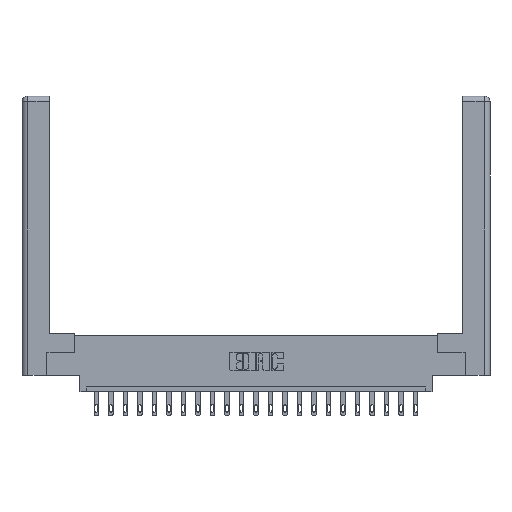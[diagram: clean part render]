
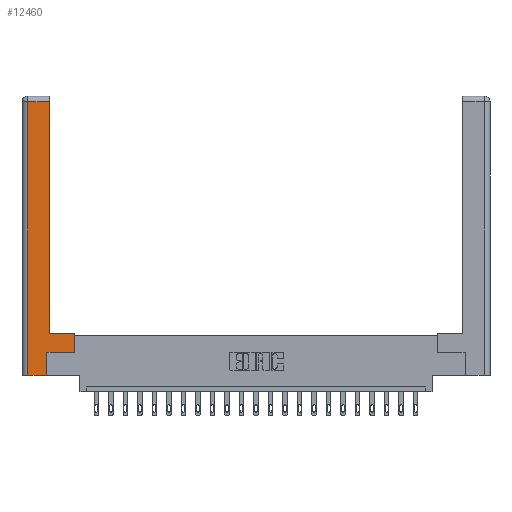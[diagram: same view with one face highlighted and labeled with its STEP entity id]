
A CAD part, top view. The second image highlights one B-rep face of the part: STEP entity #12460.
In plain terms, the highlighted planar face has unit normal (0, 0, 1).
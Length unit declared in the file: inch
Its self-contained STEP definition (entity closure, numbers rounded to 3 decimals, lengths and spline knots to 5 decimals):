
#573 = VERTEX_POINT ( 'NONE', #6281 ) ;
#1134 = EDGE_CURVE ( 'NONE', #573, #10981, #15123, .T. ) ;
#1169 = ORIENTED_EDGE ( 'NONE', *, *, #2353, .T. ) ;
#1260 = CARTESIAN_POINT ( 'NONE',  ( 0.565, 0.245, 0. ) ) ;
#1643 = DIRECTION ( 'NONE',  ( -1., 0., 0. ) ) ;
#2023 = EDGE_CURVE ( 'NONE', #16573, #2266, #4838, .T. ) ;
#2266 = VERTEX_POINT ( 'NONE', #18915 ) ;
#2353 = EDGE_CURVE ( 'NONE', #10981, #6185, #18006, .T. ) ;
#2727 = VERTEX_POINT ( 'NONE', #11609 ) ;
#2737 = LINE ( 'NONE', #16708, #15148 ) ;
#2863 = VECTOR ( 'NONE', #13536, 39.37008 ) ;
#2979 = DIRECTION ( 'NONE',  ( 1., 0., 0. ) ) ;
#3248 = CARTESIAN_POINT ( 'NONE',  ( 0.295, 3., 0. ) ) ;
#3903 = EDGE_CURVE ( 'NONE', #6185, #4155, #21936, .T. ) ;
#4155 = VERTEX_POINT ( 'NONE', #11891 ) ;
#4613 = LINE ( 'NONE', #1260, #11887 ) ;
#4628 = CARTESIAN_POINT ( 'NONE',  ( 0.295, 0.45, 0. ) ) ;
#4838 = LINE ( 'NONE', #12485, #19100 ) ;
#4889 = EDGE_LOOP ( 'NONE', ( #1169, #15297, #9282, #9683, #9627, #7358, #19312, #9690 ) ) ;
#5744 = CARTESIAN_POINT ( 'NONE',  ( 0.565, 0.45, 0. ) ) ;
#6147 = CARTESIAN_POINT ( 'NONE',  ( 0.565, 0.245, 0. ) ) ;
#6185 = VERTEX_POINT ( 'NONE', #16933 ) ;
#6281 = CARTESIAN_POINT ( 'NONE',  ( 0.565, 0.45, 0. ) ) ;
#6673 = FACE_OUTER_BOUND ( 'NONE', #4889, .T. ) ;
#6967 = CARTESIAN_POINT ( 'NONE',  ( 0.0615, 0., 0. ) ) ;
#7358 = ORIENTED_EDGE ( 'NONE', *, *, #20103, .T. ) ;
#8694 = CARTESIAN_POINT ( 'NONE',  ( 0.265, 0., 0. ) ) ;
#8705 = EDGE_CURVE ( 'NONE', #16233, #573, #19807, .T. ) ;
#9282 = ORIENTED_EDGE ( 'NONE', *, *, #16985, .T. ) ;
#9627 = ORIENTED_EDGE ( 'NONE', *, *, #2023, .T. ) ;
#9683 = ORIENTED_EDGE ( 'NONE', *, *, #19991, .T. ) ;
#9690 = ORIENTED_EDGE ( 'NONE', *, *, #1134, .T. ) ;
#9798 = CARTESIAN_POINT ( 'NONE',  ( 0.295, 0.45, 0. ) ) ;
#10948 = DIRECTION ( 'NONE',  ( 0., 1., 0. ) ) ;
#10958 = VECTOR ( 'NONE', #10948, 39.37008 ) ;
#10981 = VERTEX_POINT ( 'NONE', #9798 ) ;
#11080 = DIRECTION ( 'NONE',  ( -1., 0., 0. ) ) ;
#11609 = CARTESIAN_POINT ( 'NONE',  ( 0.0615, 0., 0. ) ) ;
#11887 = VECTOR ( 'NONE', #2979, 39.37008 ) ;
#11891 = CARTESIAN_POINT ( 'NONE',  ( 0.0615, 2.94, 0. ) ) ;
#12261 = DIRECTION ( 'NONE',  ( 0., 1., 0. ) ) ;
#12460 = ADVANCED_FACE ( 'NONE', ( #6673 ), #15360, .F. ) ;
#12485 = CARTESIAN_POINT ( 'NONE',  ( 0.265, 0.245, 0. ) ) ;
#13198 = VECTOR ( 'NONE', #15308, 39.37008 ) ;
#13536 = DIRECTION ( 'NONE',  ( 0., -1., 0. ) ) ;
#13633 = CARTESIAN_POINT ( 'NONE',  ( 0., 0., 0. ) ) ;
#15123 = LINE ( 'NONE', #4628, #19389 ) ;
#15148 = VECTOR ( 'NONE', #20046, 39.37008 ) ;
#15297 = ORIENTED_EDGE ( 'NONE', *, *, #3903, .T. ) ;
#15308 = DIRECTION ( 'NONE',  ( 0., 1., 0. ) ) ;
#15360 = PLANE ( 'NONE',  #17925 ) ;
#16072 = VECTOR ( 'NONE', #18139, 39.37008 ) ;
#16233 = VERTEX_POINT ( 'NONE', #6147 ) ;
#16573 = VERTEX_POINT ( 'NONE', #8694 ) ;
#16708 = CARTESIAN_POINT ( 'NONE',  ( 0.265, 0., 0. ) ) ;
#16933 = CARTESIAN_POINT ( 'NONE',  ( 0.295, 2.94, 0. ) ) ;
#16985 = EDGE_CURVE ( 'NONE', #4155, #2727, #21670, .T. ) ;
#17925 = AXIS2_PLACEMENT_3D ( 'NONE', #13633, #22224, #1643 ) ;
#18006 = LINE ( 'NONE', #3248, #13198 ) ;
#18139 = DIRECTION ( 'NONE',  ( -1., 0., 0. ) ) ;
#18915 = CARTESIAN_POINT ( 'NONE',  ( 0.265, 0.245, 0. ) ) ;
#19100 = VECTOR ( 'NONE', #12261, 39.37008 ) ;
#19312 = ORIENTED_EDGE ( 'NONE', *, *, #8705, .T. ) ;
#19389 = VECTOR ( 'NONE', #11080, 39.37008 ) ;
#19807 = LINE ( 'NONE', #5744, #10958 ) ;
#19991 = EDGE_CURVE ( 'NONE', #2727, #16573, #2737, .T. ) ;
#20046 = DIRECTION ( 'NONE',  ( 1., 0., 0. ) ) ;
#20103 = EDGE_CURVE ( 'NONE', #2266, #16233, #4613, .T. ) ;
#21499 = CARTESIAN_POINT ( 'NONE',  ( 0.0615, 2.94, 0. ) ) ;
#21670 = LINE ( 'NONE', #6967, #2863 ) ;
#21936 = LINE ( 'NONE', #21499, #16072 ) ;
#22224 = DIRECTION ( 'NONE',  ( 0., 0., -1. ) ) ;
